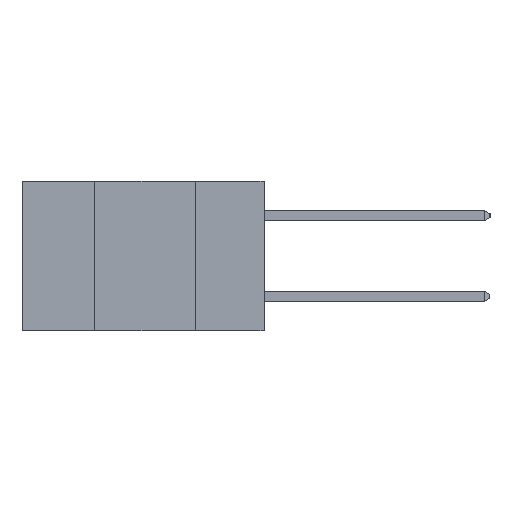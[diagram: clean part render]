
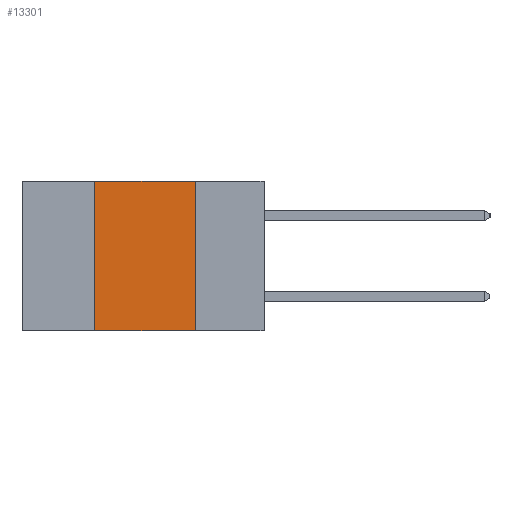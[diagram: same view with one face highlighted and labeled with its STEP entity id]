
A CAD part, left-side view. The second image highlights one B-rep face of the part: STEP entity #13301.
In plain terms, the highlighted planar face has unit normal (-1, 0, 0).
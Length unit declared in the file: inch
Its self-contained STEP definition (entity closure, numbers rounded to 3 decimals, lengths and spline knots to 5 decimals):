
#674 = VERTEX_POINT ( 'NONE', #11537 ) ;
#979 = CARTESIAN_POINT ( 'NONE',  ( 0., 0.42, -0.37 ) ) ;
#983 = LINE ( 'NONE', #8207, #12352 ) ;
#1068 = CARTESIAN_POINT ( 'NONE',  ( 0., 0.42, -0.37 ) ) ;
#1255 = VECTOR ( 'NONE', #10108, 39.37008 ) ;
#1336 = EDGE_CURVE ( 'NONE', #674, #11731, #4680, .T. ) ;
#1703 = CARTESIAN_POINT ( 'NONE',  ( 0., 0.6, 0. ) ) ;
#2880 = LINE ( 'NONE', #1703, #1255 ) ;
#3253 = DIRECTION ( 'NONE',  ( 1., 0., 0. ) ) ;
#3338 = DIRECTION ( 'NONE',  ( 0., 0., -1. ) ) ;
#3477 = ORIENTED_EDGE ( 'NONE', *, *, #12709, .F. ) ;
#3519 = EDGE_LOOP ( 'NONE', ( #8838, #3477, #8213, #9649 ) ) ;
#4331 = FACE_OUTER_BOUND ( 'NONE', #3519, .T. ) ;
#4680 = LINE ( 'NONE', #14638, #6016 ) ;
#5036 = VERTEX_POINT ( 'NONE', #9664 ) ;
#5413 = CARTESIAN_POINT ( 'NONE',  ( 0., 0.17, -0.37 ) ) ;
#5621 = VECTOR ( 'NONE', #13338, 39.37008 ) ;
#5969 = AXIS2_PLACEMENT_3D ( 'NONE', #14198, #3253, #3338 ) ;
#6016 = VECTOR ( 'NONE', #9447, 39.37008 ) ;
#7307 = LINE ( 'NONE', #1068, #5621 ) ;
#8207 = CARTESIAN_POINT ( 'NONE',  ( 0., 0.6, -0.37 ) ) ;
#8213 = ORIENTED_EDGE ( 'NONE', *, *, #9964, .F. ) ;
#8838 = ORIENTED_EDGE ( 'NONE', *, *, #1336, .F. ) ;
#9232 = EDGE_CURVE ( 'NONE', #9953, #11731, #983, .T. ) ;
#9263 = PLANE ( 'NONE',  #5969 ) ;
#9447 = DIRECTION ( 'NONE',  ( 0., 0., -1. ) ) ;
#9649 = ORIENTED_EDGE ( 'NONE', *, *, #9232, .T. ) ;
#9664 = CARTESIAN_POINT ( 'NONE',  ( 0., 0.42, 0. ) ) ;
#9953 = VERTEX_POINT ( 'NONE', #979 ) ;
#9964 = EDGE_CURVE ( 'NONE', #9953, #5036, #7307, .T. ) ;
#10108 = DIRECTION ( 'NONE',  ( 0., -1., 0. ) ) ;
#10924 = DIRECTION ( 'NONE',  ( 0., -1., 0. ) ) ;
#11537 = CARTESIAN_POINT ( 'NONE',  ( 0., 0.17, 0. ) ) ;
#11731 = VERTEX_POINT ( 'NONE', #5413 ) ;
#12352 = VECTOR ( 'NONE', #10924, 39.37008 ) ;
#12709 = EDGE_CURVE ( 'NONE', #5036, #674, #2880, .T. ) ;
#13301 = ADVANCED_FACE ( 'NONE', ( #4331 ), #9263, .F. ) ;
#13338 = DIRECTION ( 'NONE',  ( 0., 0., 1. ) ) ;
#14198 = CARTESIAN_POINT ( 'NONE',  ( 0., 0.6, 0. ) ) ;
#14638 = CARTESIAN_POINT ( 'NONE',  ( 0., 0.17, -0.37 ) ) ;
